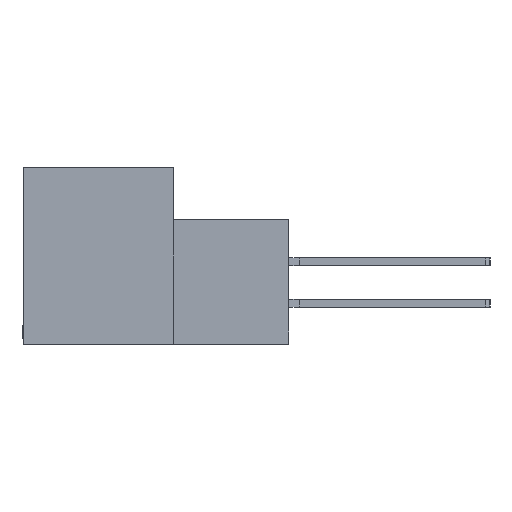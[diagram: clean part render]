
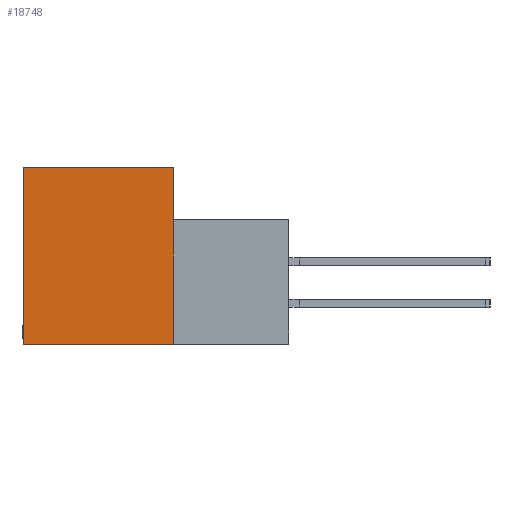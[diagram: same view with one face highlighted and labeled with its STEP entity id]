
A CAD part, left-side view. The second image highlights one B-rep face of the part: STEP entity #18748.
In plain terms, the highlighted planar face has unit normal (-1, 0, 0).
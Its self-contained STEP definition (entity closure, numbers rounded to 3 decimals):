
#918 = CARTESIAN_POINT ( 'NONE',  ( 0., 0., -13.487 ) ) ;
#1574 = FACE_OUTER_BOUND ( 'NONE', #2634, .T. ) ;
#1805 = VECTOR ( 'NONE', #6385, 1000. ) ;
#2276 = VECTOR ( 'NONE', #29124, 1000. ) ;
#2634 = EDGE_LOOP ( 'NONE', ( #17953, #26200, #20409, #10412 ) ) ;
#4272 = VERTEX_POINT ( 'NONE', #6987 ) ;
#4386 = LINE ( 'NONE', #29322, #2276 ) ;
#6005 = CARTESIAN_POINT ( 'NONE',  ( 0., 11.506, 0. ) ) ;
#6211 = EDGE_CURVE ( 'NONE', #15111, #25394, #7649, .T. ) ;
#6371 = PLANE ( 'NONE',  #20771 ) ;
#6385 = DIRECTION ( 'NONE',  ( 0., -1., 0. ) ) ;
#6987 = CARTESIAN_POINT ( 'NONE',  ( 0., 0., 0. ) ) ;
#7142 = DIRECTION ( 'NONE',  ( 0., 0., -1. ) ) ;
#7244 = EDGE_CURVE ( 'NONE', #18986, #15111, #4386, .T. ) ;
#7289 = VECTOR ( 'NONE', #25804, 1000. ) ;
#7649 = LINE ( 'NONE', #21320, #7289 ) ;
#10412 = ORIENTED_EDGE ( 'NONE', *, *, #6211, .F. ) ;
#11935 = CARTESIAN_POINT ( 'NONE',  ( 0., 11.506, -13.487 ) ) ;
#12753 = EDGE_CURVE ( 'NONE', #4272, #18986, #22629, .T. ) ;
#13780 = VECTOR ( 'NONE', #22269, 1000. ) ;
#13853 = DIRECTION ( 'NONE',  ( 1., 0., 0. ) ) ;
#15111 = VERTEX_POINT ( 'NONE', #11935 ) ;
#17953 = ORIENTED_EDGE ( 'NONE', *, *, #7244, .F. ) ;
#18748 = ADVANCED_FACE ( 'NONE', ( #1574 ), #6371, .F. ) ;
#18986 = VERTEX_POINT ( 'NONE', #918 ) ;
#20409 = ORIENTED_EDGE ( 'NONE', *, *, #24531, .F. ) ;
#20771 = AXIS2_PLACEMENT_3D ( 'NONE', #29289, #13853, #7142 ) ;
#21320 = CARTESIAN_POINT ( 'NONE',  ( 0., 11.506, -13.487 ) ) ;
#22269 = DIRECTION ( 'NONE',  ( 0., 0., -1. ) ) ;
#22365 = CARTESIAN_POINT ( 'NONE',  ( 0., 0., 0. ) ) ;
#22629 = LINE ( 'NONE', #22365, #13780 ) ;
#24531 = EDGE_CURVE ( 'NONE', #25394, #4272, #27621, .T. ) ;
#24743 = CARTESIAN_POINT ( 'NONE',  ( 0., 11.506, 0. ) ) ;
#25394 = VERTEX_POINT ( 'NONE', #24743 ) ;
#25804 = DIRECTION ( 'NONE',  ( 0., 0., 1. ) ) ;
#26200 = ORIENTED_EDGE ( 'NONE', *, *, #12753, .F. ) ;
#27621 = LINE ( 'NONE', #6005, #1805 ) ;
#29124 = DIRECTION ( 'NONE',  ( 0., 1., 0. ) ) ;
#29289 = CARTESIAN_POINT ( 'NONE',  ( 0., 0., 0. ) ) ;
#29322 = CARTESIAN_POINT ( 'NONE',  ( 0., -8.814, -13.487 ) ) ;
